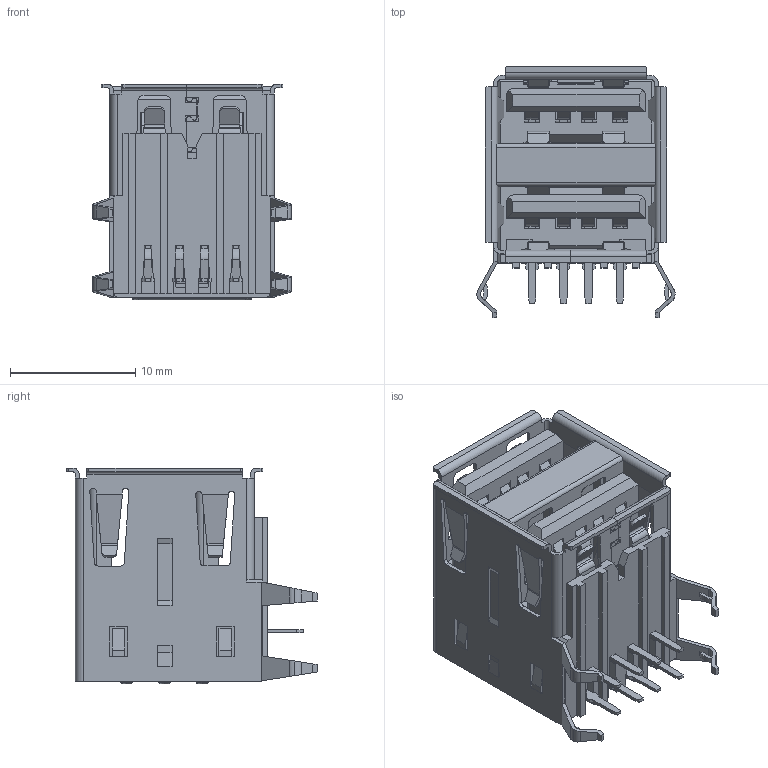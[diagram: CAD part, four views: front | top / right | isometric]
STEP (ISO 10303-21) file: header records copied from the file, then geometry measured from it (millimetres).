
FILE_DESCRIPTION (( 'STEP AP214' ), '1' );
FILE_NAME ('690N208-124-020.STEP', '2021-01-14T16:06:05', ( '' ), ( '' ), 'SwSTEP 2.0', 'SolidWorks 2020', '' );
FILE_SCHEMA (( 'AUTOMOTIVE_DESIGN' ));
Length unit declared in the file: millimetre
Products named in the file (6): Shell 2 690N208-X24-02X; Shell 690N208-X24-02X; 690N208-124-020; Insulator 690N208-X24-02X; Contact Upper 690N208-X24-02X; Contact Lower 690N208-X24-02X
Assembly tree (11 placements, depth 2):
  690N208-124-020
    Insulator 690N208-X24-02X
    Contact Lower 690N208-X24-02X  x4
    Contact Upper 690N208-X24-02X  x4
    Shell 690N208-X24-02X
    Shell 2 690N208-X24-02X
Bounding box: 15.8 x 19.98 x 17.2 mm (x, y, z)
Volume: 1553.5 mm3; surface area: 5527.1 mm2
Topology: 11 solids, 11 shells, 1766 faces, 5066 edges, 3334 vertices
Faces by surface type: plane 1394, cylinder 329, bspline 25, torus 18
Entity records: 47264 total; most frequent: CARTESIAN_POINT 9792, ORIENTED_EDGE 8152, DIRECTION 7175, EDGE_CURVE 4076, VECTOR 3325, LINE 3325, VERTEX_POINT 2674, AXIS2_PLACEMENT_3D 1925
